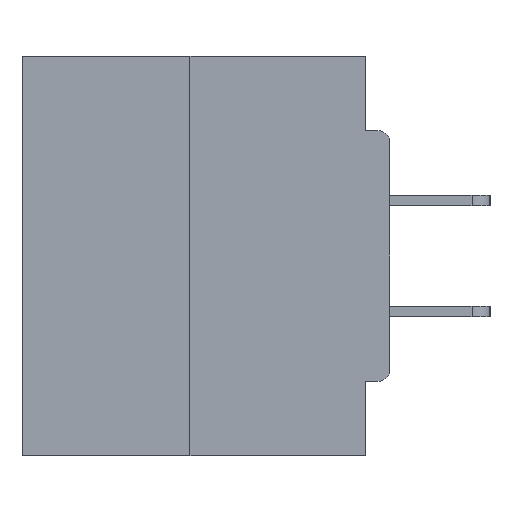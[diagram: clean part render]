
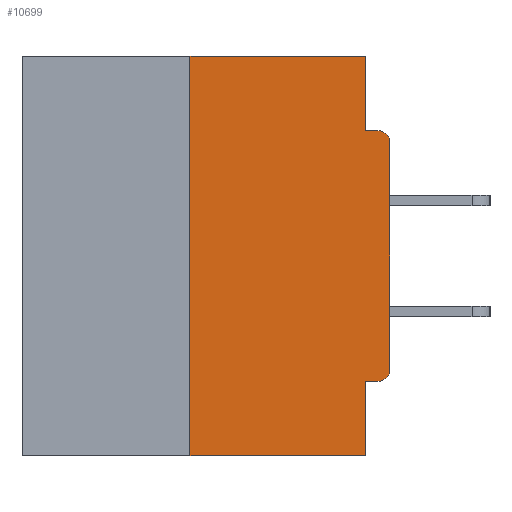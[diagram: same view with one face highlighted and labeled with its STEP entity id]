
A CAD part, left-side view. The second image highlights one B-rep face of the part: STEP entity #10699.
In plain terms, the highlighted planar face has unit normal (-1, 0, 0).
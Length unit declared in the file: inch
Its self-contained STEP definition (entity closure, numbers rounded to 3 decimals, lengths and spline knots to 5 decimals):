
#236 = EDGE_CURVE ( 'NONE', #35439, #8075, #6563, .T. ) ;
#717 = ORIENTED_EDGE ( 'NONE', *, *, #33561, .T. ) ;
#742 = VERTEX_POINT ( 'NONE', #4237 ) ;
#987 = LINE ( 'NONE', #24389, #34237 ) ;
#1009 = EDGE_CURVE ( 'NONE', #25092, #742, #30674, .T. ) ;
#1885 = CARTESIAN_POINT ( 'NONE',  ( 0., 0.015, -0.0935 ) ) ;
#2043 = VECTOR ( 'NONE', #20344, 39.37008 ) ;
#2536 = ORIENTED_EDGE ( 'NONE', *, *, #236, .F. ) ;
#2648 = DIRECTION ( 'NONE',  ( 0., -1., 0. ) ) ;
#2719 = VERTEX_POINT ( 'NONE', #23128 ) ;
#3275 = VERTEX_POINT ( 'NONE', #16561 ) ;
#3450 = CARTESIAN_POINT ( 'NONE',  ( 0., 0.031, -0.5 ) ) ;
#3798 = CARTESIAN_POINT ( 'NONE',  ( 0., 0.25, 0. ) ) ;
#4237 = CARTESIAN_POINT ( 'NONE',  ( 0., 0.031, -0.4065 ) ) ;
#4343 = ORIENTED_EDGE ( 'NONE', *, *, #8947, .T. ) ;
#4796 = VECTOR ( 'NONE', #31422, 39.37008 ) ;
#6471 = ORIENTED_EDGE ( 'NONE', *, *, #32959, .F. ) ;
#6563 = LINE ( 'NONE', #3798, #4796 ) ;
#6833 = EDGE_CURVE ( 'NONE', #25092, #2719, #18604, .T. ) ;
#7429 = EDGE_CURVE ( 'NONE', #27871, #12708, #34955, .T. ) ;
#7787 = VECTOR ( 'NONE', #2648, 39.37008 ) ;
#8032 = DIRECTION ( 'NONE',  ( 0., 0., -1. ) ) ;
#8075 = VERTEX_POINT ( 'NONE', #21671 ) ;
#8947 = EDGE_CURVE ( 'NONE', #35439, #9921, #27982, .T. ) ;
#9047 = LINE ( 'NONE', #20671, #30612 ) ;
#9253 = ORIENTED_EDGE ( 'NONE', *, *, #6833, .T. ) ;
#9262 = CARTESIAN_POINT ( 'NONE',  ( 0., 0.015, -0.4065 ) ) ;
#9921 = VERTEX_POINT ( 'NONE', #3450 ) ;
#10699 = ADVANCED_FACE ( 'NONE', ( #17569 ), #28468, .F. ) ;
#11785 = DIRECTION ( 'NONE',  ( 1., 0., 0. ) ) ;
#12708 = VERTEX_POINT ( 'NONE', #1885 ) ;
#13814 = LINE ( 'NONE', #27657, #7787 ) ;
#14099 = AXIS2_PLACEMENT_3D ( 'NONE', #15328, #23833, #18025 ) ;
#14385 = EDGE_CURVE ( 'NONE', #8075, #21118, #13814, .T. ) ;
#14533 = DIRECTION ( 'NONE',  ( 0., 0., -1. ) ) ;
#15328 = CARTESIAN_POINT ( 'NONE',  ( 0., 0.015, -0.3915 ) ) ;
#15626 = CARTESIAN_POINT ( 'NONE',  ( 0., 0., 0. ) ) ;
#15747 = EDGE_CURVE ( 'NONE', #3275, #12708, #27459, .T. ) ;
#16561 = CARTESIAN_POINT ( 'NONE',  ( 0., 0., -0.1085 ) ) ;
#16779 = ORIENTED_EDGE ( 'NONE', *, *, #20270, .F. ) ;
#16922 = ORIENTED_EDGE ( 'NONE', *, *, #15747, .T. ) ;
#17569 = FACE_OUTER_BOUND ( 'NONE', #33353, .T. ) ;
#18025 = DIRECTION ( 'NONE',  ( 0., 0., -1. ) ) ;
#18443 = DIRECTION ( 'NONE',  ( 0., 0., 1. ) ) ;
#18604 = CIRCLE ( 'NONE', #14099, 0.015 ) ;
#18701 = ORIENTED_EDGE ( 'NONE', *, *, #7429, .F. ) ;
#20270 = EDGE_CURVE ( 'NONE', #742, #9921, #9047, .T. ) ;
#20344 = DIRECTION ( 'NONE',  ( 0., -1., 0. ) ) ;
#20544 = AXIS2_PLACEMENT_3D ( 'NONE', #34102, #11785, #14533 ) ;
#20671 = CARTESIAN_POINT ( 'NONE',  ( 0., 0.031, -0.5 ) ) ;
#21118 = VERTEX_POINT ( 'NONE', #27568 ) ;
#21325 = ORIENTED_EDGE ( 'NONE', *, *, #1009, .F. ) ;
#21671 = CARTESIAN_POINT ( 'NONE',  ( 0., 0.25, 0. ) ) ;
#21968 = DIRECTION ( 'NONE',  ( 0., 1., 0. ) ) ;
#21997 = DIRECTION ( 'NONE',  ( 0., 0., -1. ) ) ;
#22487 = VECTOR ( 'NONE', #21968, 39.37008 ) ;
#23128 = CARTESIAN_POINT ( 'NONE',  ( 0., 0., -0.3915 ) ) ;
#23572 = CARTESIAN_POINT ( 'NONE',  ( 0., 0.031, -0.0935 ) ) ;
#23833 = DIRECTION ( 'NONE',  ( -1., 0., 0. ) ) ;
#24293 = CARTESIAN_POINT ( 'NONE',  ( 0., 0.015, -0.1085 ) ) ;
#24389 = CARTESIAN_POINT ( 'NONE',  ( 0., 0.031, 0. ) ) ;
#24607 = CARTESIAN_POINT ( 'NONE',  ( 0., 0., -0.4065 ) ) ;
#25092 = VERTEX_POINT ( 'NONE', #9262 ) ;
#25188 = VECTOR ( 'NONE', #18443, 39.37008 ) ;
#26217 = CARTESIAN_POINT ( 'NONE',  ( 0., 0.46, -0.5 ) ) ;
#26669 = CARTESIAN_POINT ( 'NONE',  ( 0., 0., -0.0935 ) ) ;
#27459 = CIRCLE ( 'NONE', #27753, 0.015 ) ;
#27568 = CARTESIAN_POINT ( 'NONE',  ( 0., 0.031, 0. ) ) ;
#27657 = CARTESIAN_POINT ( 'NONE',  ( 0., 0.46, 0. ) ) ;
#27753 = AXIS2_PLACEMENT_3D ( 'NONE', #24293, #35120, #8032 ) ;
#27871 = VERTEX_POINT ( 'NONE', #23572 ) ;
#27982 = LINE ( 'NONE', #26217, #2043 ) ;
#28468 = PLANE ( 'NONE',  #20544 ) ;
#29606 = ORIENTED_EDGE ( 'NONE', *, *, #14385, .F. ) ;
#30612 = VECTOR ( 'NONE', #31366, 39.37008 ) ;
#30674 = LINE ( 'NONE', #24607, #22487 ) ;
#31366 = DIRECTION ( 'NONE',  ( 0., 0., -1. ) ) ;
#31422 = DIRECTION ( 'NONE',  ( 0., 0., 1. ) ) ;
#32320 = DIRECTION ( 'NONE',  ( 0., -1., 0. ) ) ;
#32500 = LINE ( 'NONE', #15626, #25188 ) ;
#32780 = CARTESIAN_POINT ( 'NONE',  ( 0., 0.25, -0.5 ) ) ;
#32959 = EDGE_CURVE ( 'NONE', #21118, #27871, #987, .T. ) ;
#33353 = EDGE_LOOP ( 'NONE', ( #29606, #2536, #4343, #16779, #21325, #9253, #717, #16922, #18701, #6471 ) ) ;
#33561 = EDGE_CURVE ( 'NONE', #2719, #3275, #32500, .T. ) ;
#34102 = CARTESIAN_POINT ( 'NONE',  ( 0., 0.46, 0. ) ) ;
#34118 = VECTOR ( 'NONE', #32320, 39.37008 ) ;
#34237 = VECTOR ( 'NONE', #21997, 39.37008 ) ;
#34955 = LINE ( 'NONE', #26669, #34118 ) ;
#35120 = DIRECTION ( 'NONE',  ( -1., 0., 0. ) ) ;
#35439 = VERTEX_POINT ( 'NONE', #32780 ) ;
